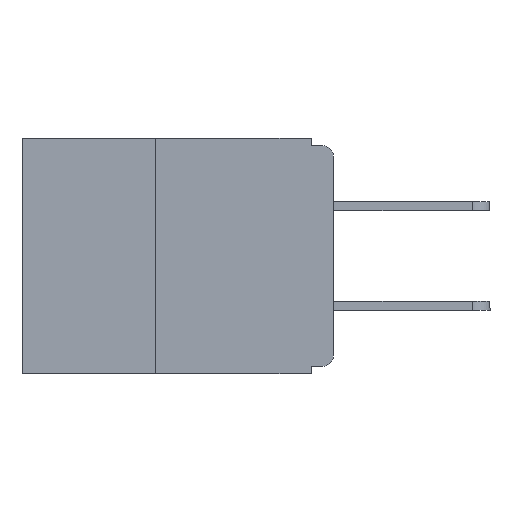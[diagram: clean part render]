
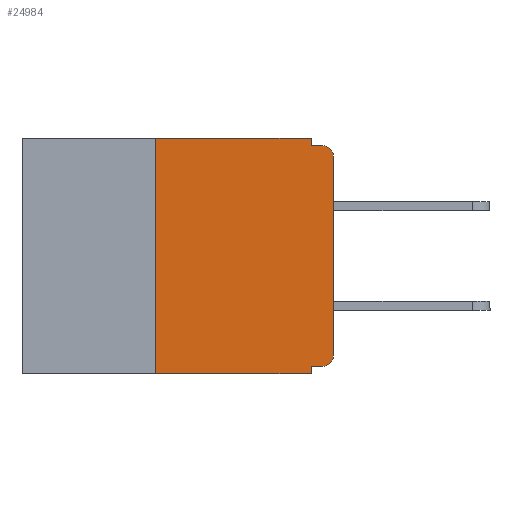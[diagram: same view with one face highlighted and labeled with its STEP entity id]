
A CAD part, left-side view. The second image highlights one B-rep face of the part: STEP entity #24984.
In plain terms, the highlighted planar face has unit normal (-1, 0, 0).
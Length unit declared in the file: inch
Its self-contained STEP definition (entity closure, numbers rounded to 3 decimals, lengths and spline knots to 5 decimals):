
#60 = VECTOR ( 'NONE', #21166, 39.37008 ) ;
#762 = CARTESIAN_POINT ( 'NONE',  ( 0., 0.437, 0. ) ) ;
#867 = VERTEX_POINT ( 'NONE', #10801 ) ;
#910 = VECTOR ( 'NONE', #2479, 39.37008 ) ;
#1834 = CARTESIAN_POINT ( 'NONE',  ( 0., 0.031, -0.33 ) ) ;
#1948 = DIRECTION ( 'NONE',  ( 0., 0., 1. ) ) ;
#2479 = DIRECTION ( 'NONE',  ( 0., 0., 1. ) ) ;
#2810 = VERTEX_POINT ( 'NONE', #22459 ) ;
#3667 = CARTESIAN_POINT ( 'NONE',  ( 0., 0.031, 0. ) ) ;
#3838 = ORIENTED_EDGE ( 'NONE', *, *, #18730, .F. ) ;
#4043 = DIRECTION ( 'NONE',  ( 0., 1., 0. ) ) ;
#4310 = FACE_OUTER_BOUND ( 'NONE', #27699, .T. ) ;
#4325 = VERTEX_POINT ( 'NONE', #16531 ) ;
#4795 = LINE ( 'NONE', #24888, #26418 ) ;
#4869 = CARTESIAN_POINT ( 'NONE',  ( 0., 0., -0.025 ) ) ;
#4888 = CARTESIAN_POINT ( 'NONE',  ( 0., 0.031, -0.33 ) ) ;
#5080 = LINE ( 'NONE', #8693, #27327 ) ;
#5479 = CARTESIAN_POINT ( 'NONE',  ( 0., 0.031, 0. ) ) ;
#5567 = ORIENTED_EDGE ( 'NONE', *, *, #7492, .T. ) ;
#6589 = EDGE_CURVE ( 'NONE', #22728, #25194, #13551, .T. ) ;
#6676 = LINE ( 'NONE', #22937, #17582 ) ;
#7014 = LINE ( 'NONE', #13550, #910 ) ;
#7492 = EDGE_CURVE ( 'NONE', #19640, #7507, #7014, .T. ) ;
#7507 = VERTEX_POINT ( 'NONE', #4869 ) ;
#7659 = DIRECTION ( 'NONE',  ( 0., -1., 0. ) ) ;
#7760 = VECTOR ( 'NONE', #4043, 39.37008 ) ;
#7913 = EDGE_CURVE ( 'NONE', #22728, #19640, #19908, .T. ) ;
#8693 = CARTESIAN_POINT ( 'NONE',  ( 0., 0.25, -0.33 ) ) ;
#8859 = CARTESIAN_POINT ( 'NONE',  ( 0., 0.015, -0.01 ) ) ;
#9426 = VERTEX_POINT ( 'NONE', #8859 ) ;
#9950 = DIRECTION ( 'NONE',  ( -1., 0., 0. ) ) ;
#10110 = ORIENTED_EDGE ( 'NONE', *, *, #6589, .F. ) ;
#10514 = CARTESIAN_POINT ( 'NONE',  ( 0., 0.437, 0. ) ) ;
#10801 = CARTESIAN_POINT ( 'NONE',  ( 0., 0.031, -0.01 ) ) ;
#10925 = EDGE_CURVE ( 'NONE', #2810, #4325, #5080, .T. ) ;
#11803 = ORIENTED_EDGE ( 'NONE', *, *, #16744, .T. ) ;
#12008 = LINE ( 'NONE', #3667, #60 ) ;
#12962 = CARTESIAN_POINT ( 'NONE',  ( 0., 0.015, -0.305 ) ) ;
#13550 = CARTESIAN_POINT ( 'NONE',  ( 0., 0., 0. ) ) ;
#13551 = LINE ( 'NONE', #15010, #7760 ) ;
#14122 = DIRECTION ( 'NONE',  ( 0., -1., 0. ) ) ;
#14363 = VECTOR ( 'NONE', #23686, 39.37008 ) ;
#14364 = DIRECTION ( 'NONE',  ( 0., -1., 0. ) ) ;
#14876 = DIRECTION ( 'NONE',  ( 0., 0., -1. ) ) ;
#15010 = CARTESIAN_POINT ( 'NONE',  ( 0., 0., -0.32 ) ) ;
#15036 = LINE ( 'NONE', #1834, #14363 ) ;
#15125 = DIRECTION ( 'NONE',  ( 0., 0., -1. ) ) ;
#15923 = VECTOR ( 'NONE', #14122, 39.37008 ) ;
#16201 = ORIENTED_EDGE ( 'NONE', *, *, #25802, .F. ) ;
#16531 = CARTESIAN_POINT ( 'NONE',  ( 0., 0.25, 0. ) ) ;
#16744 = EDGE_CURVE ( 'NONE', #2810, #17730, #6676, .T. ) ;
#17382 = VERTEX_POINT ( 'NONE', #5479 ) ;
#17582 = VECTOR ( 'NONE', #14364, 39.37008 ) ;
#17730 = VERTEX_POINT ( 'NONE', #4888 ) ;
#17894 = EDGE_CURVE ( 'NONE', #867, #9426, #4795, .T. ) ;
#18730 = EDGE_CURVE ( 'NONE', #17382, #867, #12008, .T. ) ;
#19196 = EDGE_CURVE ( 'NONE', #7507, #9426, #26975, .T. ) ;
#19450 = CARTESIAN_POINT ( 'NONE',  ( 0., 0., -0.305 ) ) ;
#19628 = ORIENTED_EDGE ( 'NONE', *, *, #23926, .F. ) ;
#19640 = VERTEX_POINT ( 'NONE', #19450 ) ;
#19908 = CIRCLE ( 'NONE', #26382, 0.015 ) ;
#20110 = AXIS2_PLACEMENT_3D ( 'NONE', #10514, #27584, #14876 ) ;
#20611 = ORIENTED_EDGE ( 'NONE', *, *, #17894, .F. ) ;
#21166 = DIRECTION ( 'NONE',  ( 0., 0., -1. ) ) ;
#21624 = CARTESIAN_POINT ( 'NONE',  ( 0., 0.015, -0.32 ) ) ;
#22303 = ORIENTED_EDGE ( 'NONE', *, *, #7913, .T. ) ;
#22459 = CARTESIAN_POINT ( 'NONE',  ( 0., 0.25, -0.33 ) ) ;
#22728 = VERTEX_POINT ( 'NONE', #21624 ) ;
#22734 = CARTESIAN_POINT ( 'NONE',  ( 0., 0.031, -0.32 ) ) ;
#22903 = CARTESIAN_POINT ( 'NONE',  ( 0., 0.015, -0.025 ) ) ;
#22937 = CARTESIAN_POINT ( 'NONE',  ( 0., 0.437, -0.33 ) ) ;
#22938 = ORIENTED_EDGE ( 'NONE', *, *, #19196, .T. ) ;
#23455 = PLANE ( 'NONE',  #20110 ) ;
#23686 = DIRECTION ( 'NONE',  ( 0., 0., -1. ) ) ;
#23926 = EDGE_CURVE ( 'NONE', #25194, #17730, #15036, .T. ) ;
#24888 = CARTESIAN_POINT ( 'NONE',  ( 0., 0., -0.01 ) ) ;
#24984 = ADVANCED_FACE ( 'NONE', ( #4310 ), #23455, .F. ) ;
#24990 = DIRECTION ( 'NONE',  ( 0., 0., -1. ) ) ;
#25194 = VERTEX_POINT ( 'NONE', #22734 ) ;
#25802 = EDGE_CURVE ( 'NONE', #4325, #17382, #26548, .T. ) ;
#26382 = AXIS2_PLACEMENT_3D ( 'NONE', #12962, #27832, #15125 ) ;
#26418 = VECTOR ( 'NONE', #7659, 39.37008 ) ;
#26548 = LINE ( 'NONE', #762, #15923 ) ;
#26975 = CIRCLE ( 'NONE', #27877, 0.015 ) ;
#27327 = VECTOR ( 'NONE', #1948, 39.37008 ) ;
#27584 = DIRECTION ( 'NONE',  ( 1., 0., 0. ) ) ;
#27699 = EDGE_LOOP ( 'NONE', ( #5567, #22938, #20611, #3838, #16201, #28132, #11803, #19628, #10110, #22303 ) ) ;
#27832 = DIRECTION ( 'NONE',  ( -1., 0., 0. ) ) ;
#27877 = AXIS2_PLACEMENT_3D ( 'NONE', #22903, #9950, #24990 ) ;
#28132 = ORIENTED_EDGE ( 'NONE', *, *, #10925, .F. ) ;
